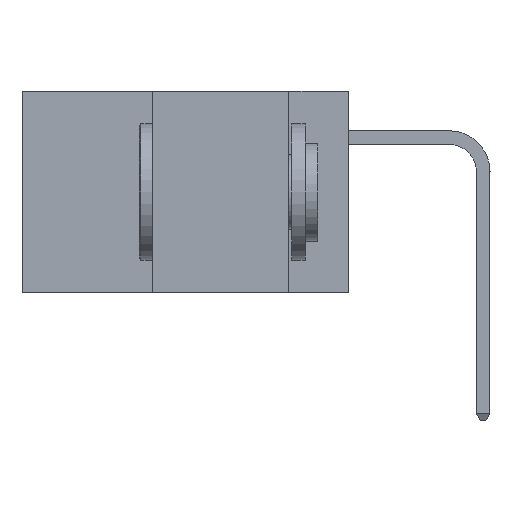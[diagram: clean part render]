
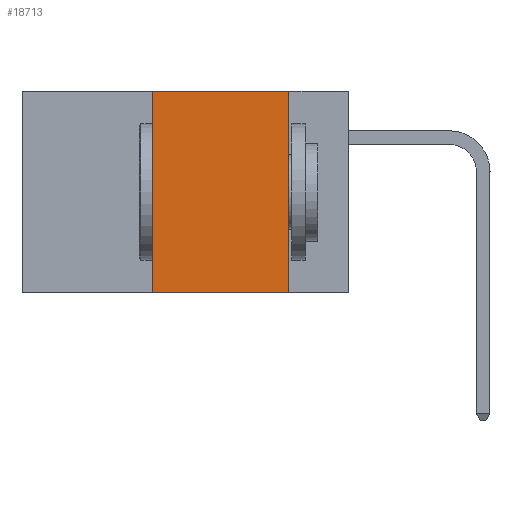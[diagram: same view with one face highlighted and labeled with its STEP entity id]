
A CAD part, left-side view. The second image highlights one B-rep face of the part: STEP entity #18713.
In plain terms, the highlighted planar face has unit normal (-1, 0, 0).
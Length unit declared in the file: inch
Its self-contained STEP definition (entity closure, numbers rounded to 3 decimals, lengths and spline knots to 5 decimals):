
#269 = DIRECTION ( 'NONE',  ( 0., -1., 0. ) ) ;
#751 = EDGE_CURVE ( 'NONE', #3935, #8267, #26759, .T. ) ;
#1536 = ORIENTED_EDGE ( 'NONE', *, *, #16867, .T. ) ;
#2290 = DIRECTION ( 'NONE',  ( 0., -1., 0. ) ) ;
#2434 = DIRECTION ( 'NONE',  ( 1., 0., 0. ) ) ;
#2732 = DIRECTION ( 'NONE',  ( 0., 0., -1. ) ) ;
#2904 = ORIENTED_EDGE ( 'NONE', *, *, #5217, .F. ) ;
#3935 = VERTEX_POINT ( 'NONE', #11174 ) ;
#5217 = EDGE_CURVE ( 'NONE', #30844, #32176, #27234, .T. ) ;
#5455 = VECTOR ( 'NONE', #15351, 39.37008 ) ;
#7175 = CARTESIAN_POINT ( 'NONE',  ( 0., 0.11, 0. ) ) ;
#7486 = VECTOR ( 'NONE', #2290, 39.37008 ) ;
#8267 = VERTEX_POINT ( 'NONE', #18141 ) ;
#8407 = LINE ( 'NONE', #36721, #7486 ) ;
#9027 = CARTESIAN_POINT ( 'NONE',  ( 0., 0.6, 0. ) ) ;
#11174 = CARTESIAN_POINT ( 'NONE',  ( 0., 0.36, -0.37 ) ) ;
#11609 = CARTESIAN_POINT ( 'NONE',  ( 0., 0.11, 0. ) ) ;
#14368 = ORIENTED_EDGE ( 'NONE', *, *, #751, .F. ) ;
#14694 = FACE_OUTER_BOUND ( 'NONE', #31133, .T. ) ;
#15351 = DIRECTION ( 'NONE',  ( 0., 0., 1. ) ) ;
#15459 = CARTESIAN_POINT ( 'NONE',  ( 0., 0.36, 0. ) ) ;
#16867 = EDGE_CURVE ( 'NONE', #3935, #32176, #8407, .T. ) ;
#18141 = CARTESIAN_POINT ( 'NONE',  ( 0., 0.36, 0. ) ) ;
#18713 = ADVANCED_FACE ( 'NONE', ( #14694 ), #36731, .F. ) ;
#19653 = CARTESIAN_POINT ( 'NONE',  ( 0., 0.11, -0.37 ) ) ;
#20247 = ORIENTED_EDGE ( 'NONE', *, *, #28149, .F. ) ;
#22776 = DIRECTION ( 'NONE',  ( 0., 0., -1. ) ) ;
#26759 = LINE ( 'NONE', #15459, #5455 ) ;
#27234 = LINE ( 'NONE', #11609, #33789 ) ;
#28149 = EDGE_CURVE ( 'NONE', #8267, #30844, #28531, .T. ) ;
#28531 = LINE ( 'NONE', #9027, #35961 ) ;
#29847 = AXIS2_PLACEMENT_3D ( 'NONE', #31267, #2434, #22776 ) ;
#30844 = VERTEX_POINT ( 'NONE', #7175 ) ;
#31133 = EDGE_LOOP ( 'NONE', ( #2904, #20247, #14368, #1536 ) ) ;
#31267 = CARTESIAN_POINT ( 'NONE',  ( 0., 0.6, 0. ) ) ;
#32176 = VERTEX_POINT ( 'NONE', #19653 ) ;
#33789 = VECTOR ( 'NONE', #2732, 39.37008 ) ;
#35961 = VECTOR ( 'NONE', #269, 39.37008 ) ;
#36721 = CARTESIAN_POINT ( 'NONE',  ( 0., 0.6, -0.37 ) ) ;
#36731 = PLANE ( 'NONE',  #29847 ) ;
